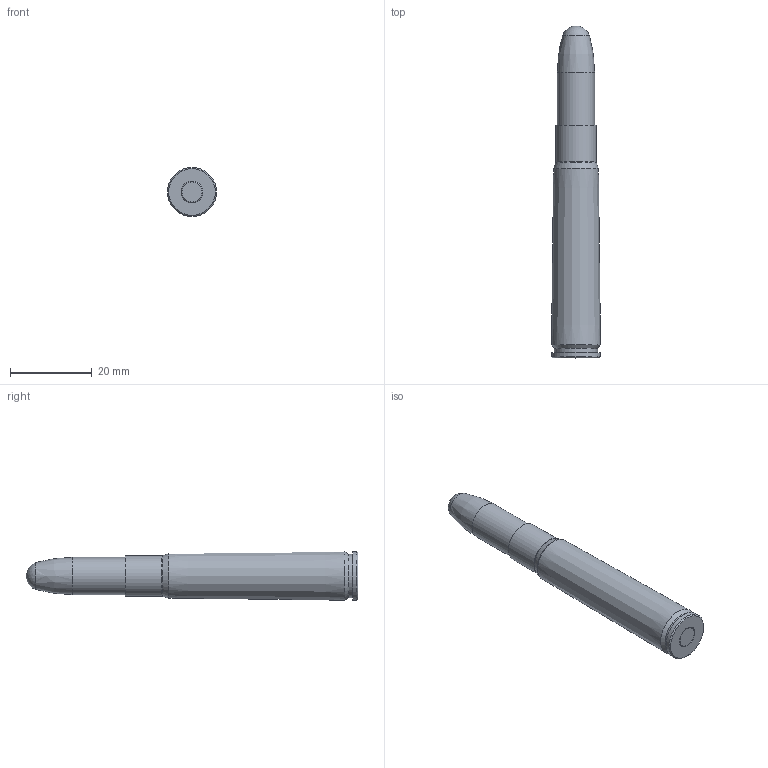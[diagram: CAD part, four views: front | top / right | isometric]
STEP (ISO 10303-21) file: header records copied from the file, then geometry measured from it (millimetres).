
FILE_DESCRIPTION((''),'2;1');
FILE_NAME('9 X 57mm Mauser.stp','2013-03-26T17:37:48',('agarrett'),(''),'Autodesk Inventor 2012','Autodesk Inventor 2012','');
FILE_SCHEMA(('AUTOMOTIVE_DESIGN { 1 0 10303 214 1 1 1 1 }'));
Length unit declared in the file: inch
Products named in the file (4): Rimless Bottleneck Assembly; Rimless Bottleneck; SpitzerPoint; PRIMER
Assembly tree (3 placements, depth 2):
  Rimless Bottleneck Assembly
    Rimless Bottleneck
    SpitzerPoint
    PRIMER
Bounding box: 11.95 x 80.98 x 11.95 mm (x, y, z)
Volume: 3680.8 mm3; surface area: 5438.3 mm2
Topology: 3 solids, 3 shells, 34 faces, 56 edges, 32 vertices
Faces by surface type: cylinder 9, plane 9, torus 8, cone 6, bspline 1, sphere 1
Full cylindrical faces by diameter (mm): 1.778 x1, 5.08 x1, 5.334 x2, 9.081 x2, 9.83 x1, 10.5 x1, 11.951 x1
Entity records: 824 total; most frequent: DIRECTION 144, CARTESIAN_POINT 131, AXIS2_PLACEMENT_3D 72, ORIENTED_EDGE 64, EDGE_LOOP 64, FACE_OUTER_BOUND 34, ADVANCED_FACE 34, VERTEX_POINT 32
